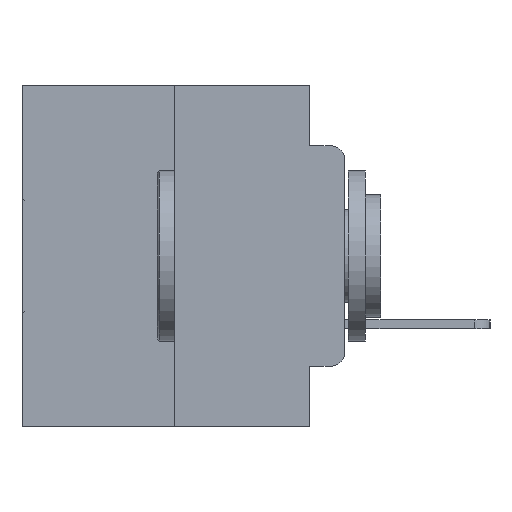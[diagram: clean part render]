
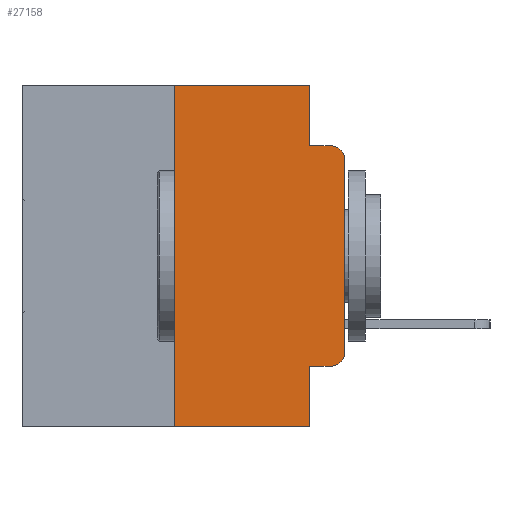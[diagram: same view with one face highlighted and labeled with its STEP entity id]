
A CAD part, left-side view. The second image highlights one B-rep face of the part: STEP entity #27158.
In plain terms, the highlighted planar face has unit normal (-1, 0, 0).
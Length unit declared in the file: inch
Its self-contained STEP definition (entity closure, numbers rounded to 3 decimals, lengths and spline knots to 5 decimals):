
#16 = VERTEX_POINT ( 'NONE', #3238 ) ;
#62 = CARTESIAN_POINT ( 'NONE',  ( 0., 0.051, 0. ) ) ;
#836 = CARTESIAN_POINT ( 'NONE',  ( 0., 0., 0. ) ) ;
#883 = EDGE_CURVE ( 'NONE', #10409, #20949, #21277, .T. ) ;
#2884 = ORIENTED_EDGE ( 'NONE', *, *, #21837, .T. ) ;
#3235 = VERTEX_POINT ( 'NONE', #62 ) ;
#3238 = CARTESIAN_POINT ( 'NONE',  ( 0., 0.02, -0.0885 ) ) ;
#3477 = VECTOR ( 'NONE', #21278, 39.37008 ) ;
#3481 = VECTOR ( 'NONE', #20890, 39.37008 ) ;
#3489 = VERTEX_POINT ( 'NONE', #16718 ) ;
#3814 = VECTOR ( 'NONE', #17365, 39.37008 ) ;
#3935 = EDGE_CURVE ( 'NONE', #10409, #12911, #10400, .T. ) ;
#4001 = ORIENTED_EDGE ( 'NONE', *, *, #3935, .F. ) ;
#4396 = ORIENTED_EDGE ( 'NONE', *, *, #23189, .F. ) ;
#4766 = ORIENTED_EDGE ( 'NONE', *, *, #9250, .T. ) ;
#4783 = DIRECTION ( 'NONE',  ( 0., 0., 1. ) ) ;
#5941 = CARTESIAN_POINT ( 'NONE',  ( 0., 0.25, -0.5 ) ) ;
#6962 = EDGE_CURVE ( 'NONE', #23415, #8427, #13029, .T. ) ;
#7677 = DIRECTION ( 'NONE',  ( -1., 0., 0. ) ) ;
#8427 = VERTEX_POINT ( 'NONE', #23318 ) ;
#8445 = CARTESIAN_POINT ( 'NONE',  ( 0., 0.473, -0.5 ) ) ;
#8620 = VECTOR ( 'NONE', #24200, 39.37008 ) ;
#8705 = CARTESIAN_POINT ( 'NONE',  ( 0., 0.051, 0. ) ) ;
#8866 = DIRECTION ( 'NONE',  ( -1., 0., 0. ) ) ;
#9250 = EDGE_CURVE ( 'NONE', #23415, #12911, #17775, .T. ) ;
#10019 = EDGE_CURVE ( 'NONE', #3235, #3489, #20435, .T. ) ;
#10239 = AXIS2_PLACEMENT_3D ( 'NONE', #20983, #7677, #23168 ) ;
#10243 = LINE ( 'NONE', #836, #3481 ) ;
#10314 = CARTESIAN_POINT ( 'NONE',  ( 0., 0., -0.1085 ) ) ;
#10400 = LINE ( 'NONE', #26966, #17704 ) ;
#10409 = VERTEX_POINT ( 'NONE', #27765 ) ;
#11741 = ORIENTED_EDGE ( 'NONE', *, *, #10019, .F. ) ;
#12450 = LINE ( 'NONE', #20633, #23443 ) ;
#12566 = DIRECTION ( 'NONE',  ( 1., 0., 0. ) ) ;
#12891 = AXIS2_PLACEMENT_3D ( 'NONE', #21294, #12566, #27839 ) ;
#12911 = VERTEX_POINT ( 'NONE', #19547 ) ;
#13029 = LINE ( 'NONE', #15960, #18196 ) ;
#13072 = FACE_OUTER_BOUND ( 'NONE', #27553, .T. ) ;
#13520 = CARTESIAN_POINT ( 'NONE',  ( 0., 0., -0.3915 ) ) ;
#13883 = DIRECTION ( 'NONE',  ( 0., 0., -1. ) ) ;
#15274 = CIRCLE ( 'NONE', #10239, 0.02 ) ;
#15575 = ORIENTED_EDGE ( 'NONE', *, *, #15983, .F. ) ;
#15960 = CARTESIAN_POINT ( 'NONE',  ( 0., 0.25, 0. ) ) ;
#15961 = ORIENTED_EDGE ( 'NONE', *, *, #883, .T. ) ;
#15983 = EDGE_CURVE ( 'NONE', #3489, #16, #21575, .T. ) ;
#16718 = CARTESIAN_POINT ( 'NONE',  ( 0., 0.051, -0.0885 ) ) ;
#16724 = CARTESIAN_POINT ( 'NONE',  ( 0., 0.051, -0.4115 ) ) ;
#16893 = AXIS2_PLACEMENT_3D ( 'NONE', #22118, #8866, #24358 ) ;
#17356 = DIRECTION ( 'NONE',  ( 0., -1., 0. ) ) ;
#17365 = DIRECTION ( 'NONE',  ( 0., -1., 0. ) ) ;
#17704 = VECTOR ( 'NONE', #13883, 39.37008 ) ;
#17775 = LINE ( 'NONE', #8445, #23588 ) ;
#18196 = VECTOR ( 'NONE', #4783, 39.37008 ) ;
#18823 = VERTEX_POINT ( 'NONE', #13520 ) ;
#19547 = CARTESIAN_POINT ( 'NONE',  ( 0., 0.051, -0.5 ) ) ;
#19764 = CIRCLE ( 'NONE', #16893, 0.02 ) ;
#20435 = LINE ( 'NONE', #8705, #8620 ) ;
#20633 = CARTESIAN_POINT ( 'NONE',  ( 0., 0.473, 0. ) ) ;
#20890 = DIRECTION ( 'NONE',  ( 0., 0., 1. ) ) ;
#20949 = VERTEX_POINT ( 'NONE', #26418 ) ;
#20983 = CARTESIAN_POINT ( 'NONE',  ( 0., 0.02, -0.3915 ) ) ;
#21277 = LINE ( 'NONE', #16724, #3477 ) ;
#21278 = DIRECTION ( 'NONE',  ( 0., -1., 0. ) ) ;
#21294 = CARTESIAN_POINT ( 'NONE',  ( 0., 0.473, 0. ) ) ;
#21575 = LINE ( 'NONE', #28179, #3814 ) ;
#21837 = EDGE_CURVE ( 'NONE', #24314, #16, #19764, .T. ) ;
#22118 = CARTESIAN_POINT ( 'NONE',  ( 0., 0.02, -0.1085 ) ) ;
#22456 = ORIENTED_EDGE ( 'NONE', *, *, #25347, .T. ) ;
#22922 = DIRECTION ( 'NONE',  ( 0., -1., 0. ) ) ;
#23168 = DIRECTION ( 'NONE',  ( 0., 0., -1. ) ) ;
#23189 = EDGE_CURVE ( 'NONE', #8427, #3235, #12450, .T. ) ;
#23318 = CARTESIAN_POINT ( 'NONE',  ( 0., 0.25, 0. ) ) ;
#23415 = VERTEX_POINT ( 'NONE', #5941 ) ;
#23443 = VECTOR ( 'NONE', #22922, 39.37008 ) ;
#23506 = PLANE ( 'NONE',  #12891 ) ;
#23588 = VECTOR ( 'NONE', #17356, 39.37008 ) ;
#24200 = DIRECTION ( 'NONE',  ( 0., 0., -1. ) ) ;
#24314 = VERTEX_POINT ( 'NONE', #10314 ) ;
#24358 = DIRECTION ( 'NONE',  ( 0., 0., -1. ) ) ;
#25181 = ORIENTED_EDGE ( 'NONE', *, *, #27682, .T. ) ;
#25347 = EDGE_CURVE ( 'NONE', #20949, #18823, #15274, .T. ) ;
#26418 = CARTESIAN_POINT ( 'NONE',  ( 0., 0.02, -0.4115 ) ) ;
#26916 = ORIENTED_EDGE ( 'NONE', *, *, #6962, .F. ) ;
#26966 = CARTESIAN_POINT ( 'NONE',  ( 0., 0.051, 0. ) ) ;
#27158 = ADVANCED_FACE ( 'NONE', ( #13072 ), #23506, .F. ) ;
#27553 = EDGE_LOOP ( 'NONE', ( #25181, #2884, #15575, #11741, #4396, #26916, #4766, #4001, #15961, #22456 ) ) ;
#27682 = EDGE_CURVE ( 'NONE', #18823, #24314, #10243, .T. ) ;
#27765 = CARTESIAN_POINT ( 'NONE',  ( 0., 0.051, -0.4115 ) ) ;
#27839 = DIRECTION ( 'NONE',  ( 0., 0., -1. ) ) ;
#28179 = CARTESIAN_POINT ( 'NONE',  ( 0., 0.051, -0.0885 ) ) ;
